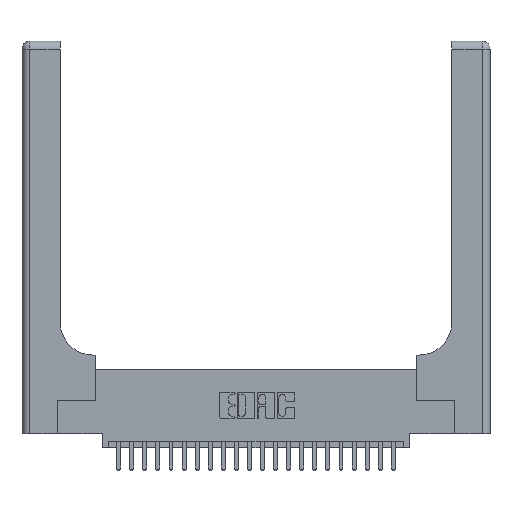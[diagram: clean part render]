
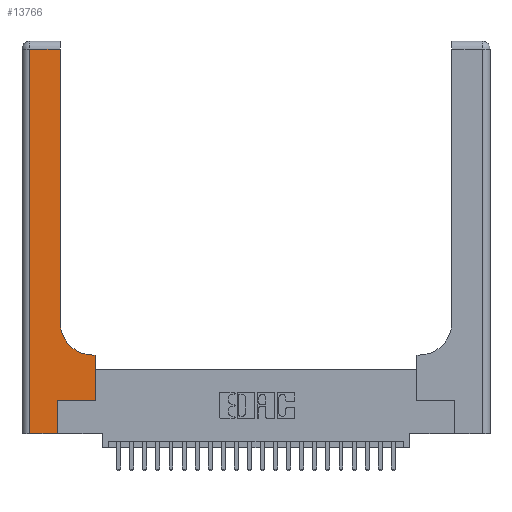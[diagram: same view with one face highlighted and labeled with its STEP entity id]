
A CAD part, top view. The second image highlights one B-rep face of the part: STEP entity #13766.
In plain terms, the highlighted planar face has unit normal (0, 0, 1).
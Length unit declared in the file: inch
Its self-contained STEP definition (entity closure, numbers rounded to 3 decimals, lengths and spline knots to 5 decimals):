
#341 = VERTEX_POINT ( 'NONE', #434 ) ;
#352 = ORIENTED_EDGE ( 'NONE', *, *, #6801, .T. ) ;
#434 = CARTESIAN_POINT ( 'NONE',  ( 0.5585, 0.6, 0.37 ) ) ;
#445 = DIRECTION ( 'NONE',  ( 1., 0., 0. ) ) ;
#485 = CARTESIAN_POINT ( 'NONE',  ( 0.2915, 3., 0.37 ) ) ;
#889 = CARTESIAN_POINT ( 'NONE',  ( 0., 3., 0.37 ) ) ;
#1382 = VECTOR ( 'NONE', #5268, 39.37008 ) ;
#1403 = VERTEX_POINT ( 'NONE', #8167 ) ;
#1989 = CARTESIAN_POINT ( 'NONE',  ( 0.269, 0., 0.37 ) ) ;
#2402 = CARTESIAN_POINT ( 'NONE',  ( 0.269, 0.25, 0.37 ) ) ;
#2750 = EDGE_CURVE ( 'NONE', #4292, #14013, #13840, .T. ) ;
#2870 = DIRECTION ( 'NONE',  ( -1., 0., 0. ) ) ;
#2989 = EDGE_CURVE ( 'NONE', #341, #19059, #18784, .T. ) ;
#3204 = VECTOR ( 'NONE', #12422, 39.37008 ) ;
#3273 = FACE_OUTER_BOUND ( 'NONE', #5727, .T. ) ;
#3636 = CARTESIAN_POINT ( 'NONE',  ( 0.5585, 0.25, 0.37 ) ) ;
#4292 = VERTEX_POINT ( 'NONE', #12453 ) ;
#4426 = CARTESIAN_POINT ( 'NONE',  ( 0.5585, 0.25, 0.37 ) ) ;
#4750 = PLANE ( 'NONE',  #5302 ) ;
#5162 = CARTESIAN_POINT ( 'NONE',  ( 0.5415, 0.85, 0.37 ) ) ;
#5268 = DIRECTION ( 'NONE',  ( 1., 0., 0. ) ) ;
#5302 = AXIS2_PLACEMENT_3D ( 'NONE', #889, #14637, #2870 ) ;
#5727 = EDGE_LOOP ( 'NONE', ( #24028, #352, #13340, #15290, #9855, #20884, #8121, #9913, #21935 ) ) ;
#5768 = CARTESIAN_POINT ( 'NONE',  ( 0.2915, 2.94, 0.37 ) ) ;
#6384 = DIRECTION ( 'NONE',  ( 0., 1., 0. ) ) ;
#6801 = EDGE_CURVE ( 'NONE', #14013, #18513, #24102, .T. ) ;
#6811 = CARTESIAN_POINT ( 'NONE',  ( 0., 2.94, 0.37 ) ) ;
#6938 = EDGE_CURVE ( 'NONE', #19831, #16864, #22894, .T. ) ;
#7126 = DIRECTION ( 'NONE',  ( 1., 0., 0. ) ) ;
#8121 = ORIENTED_EDGE ( 'NONE', *, *, #18154, .T. ) ;
#8167 = CARTESIAN_POINT ( 'NONE',  ( 0.06, 0., 0.37 ) ) ;
#8189 = AXIS2_PLACEMENT_3D ( 'NONE', #5162, #18940, #7126 ) ;
#8432 = VECTOR ( 'NONE', #18631, 39.37008 ) ;
#8519 = DIRECTION ( 'NONE',  ( 0., -1., 0. ) ) ;
#9113 = EDGE_CURVE ( 'NONE', #19059, #4292, #15415, .T. ) ;
#9855 = ORIENTED_EDGE ( 'NONE', *, *, #15202, .T. ) ;
#9913 = ORIENTED_EDGE ( 'NONE', *, *, #2989, .T. ) ;
#9957 = CARTESIAN_POINT ( 'NONE',  ( 0.06, 2.94, 0.37 ) ) ;
#10098 = CARTESIAN_POINT ( 'NONE',  ( 0.269, 0., 0.37 ) ) ;
#10986 = CARTESIAN_POINT ( 'NONE',  ( 0.2915, 0.6, 0.37 ) ) ;
#12422 = DIRECTION ( 'NONE',  ( 0., 1., 0. ) ) ;
#12453 = CARTESIAN_POINT ( 'NONE',  ( 0.2915, 0.85, 0.37 ) ) ;
#13039 = LINE ( 'NONE', #20317, #23474 ) ;
#13340 = ORIENTED_EDGE ( 'NONE', *, *, #15218, .T. ) ;
#13766 = ADVANCED_FACE ( 'NONE', ( #3273 ), #4750, .F. ) ;
#13840 = LINE ( 'NONE', #485, #17862 ) ;
#14013 = VERTEX_POINT ( 'NONE', #5768 ) ;
#14637 = DIRECTION ( 'NONE',  ( 0., 0., -1. ) ) ;
#14769 = VECTOR ( 'NONE', #24663, 39.37008 ) ;
#15202 = EDGE_CURVE ( 'NONE', #23253, #19831, #18914, .T. ) ;
#15218 = EDGE_CURVE ( 'NONE', #18513, #1403, #13039, .T. ) ;
#15290 = ORIENTED_EDGE ( 'NONE', *, *, #24567, .T. ) ;
#15415 = CIRCLE ( 'NONE', #8189, 0.25 ) ;
#15513 = LINE ( 'NONE', #23940, #24683 ) ;
#16864 = VERTEX_POINT ( 'NONE', #3636 ) ;
#17083 = CARTESIAN_POINT ( 'NONE',  ( 0.269, 0.25, 0.37 ) ) ;
#17460 = VECTOR ( 'NONE', #6384, 39.37008 ) ;
#17862 = VECTOR ( 'NONE', #20168, 39.37008 ) ;
#18064 = LINE ( 'NONE', #4426, #17460 ) ;
#18154 = EDGE_CURVE ( 'NONE', #16864, #341, #18064, .T. ) ;
#18513 = VERTEX_POINT ( 'NONE', #9957 ) ;
#18631 = DIRECTION ( 'NONE',  ( -1., 0., 0. ) ) ;
#18784 = LINE ( 'NONE', #10986, #14769 ) ;
#18914 = LINE ( 'NONE', #10098, #3204 ) ;
#18940 = DIRECTION ( 'NONE',  ( 0., 0., -1. ) ) ;
#19059 = VERTEX_POINT ( 'NONE', #23718 ) ;
#19831 = VERTEX_POINT ( 'NONE', #2402 ) ;
#20168 = DIRECTION ( 'NONE',  ( 0., 1., 0. ) ) ;
#20317 = CARTESIAN_POINT ( 'NONE',  ( 0.06, 3., 0.37 ) ) ;
#20884 = ORIENTED_EDGE ( 'NONE', *, *, #6938, .T. ) ;
#21935 = ORIENTED_EDGE ( 'NONE', *, *, #9113, .T. ) ;
#22894 = LINE ( 'NONE', #17083, #1382 ) ;
#23253 = VERTEX_POINT ( 'NONE', #1989 ) ;
#23474 = VECTOR ( 'NONE', #8519, 39.37008 ) ;
#23718 = CARTESIAN_POINT ( 'NONE',  ( 0.5415, 0.6, 0.37 ) ) ;
#23940 = CARTESIAN_POINT ( 'NONE',  ( 0., 0., 0.37 ) ) ;
#24028 = ORIENTED_EDGE ( 'NONE', *, *, #2750, .T. ) ;
#24102 = LINE ( 'NONE', #6811, #8432 ) ;
#24567 = EDGE_CURVE ( 'NONE', #1403, #23253, #15513, .T. ) ;
#24663 = DIRECTION ( 'NONE',  ( -1., 0., 0. ) ) ;
#24683 = VECTOR ( 'NONE', #445, 39.37008 ) ;
